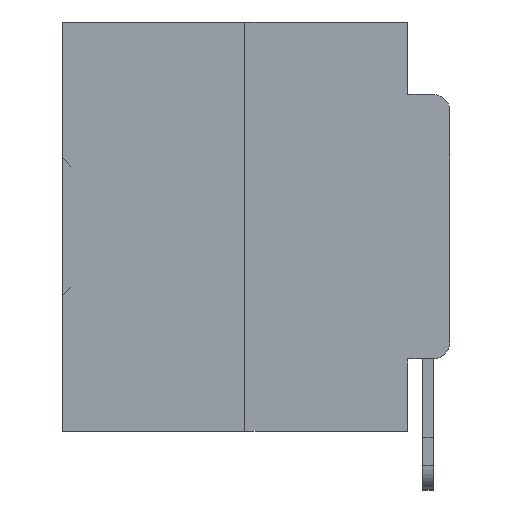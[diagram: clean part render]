
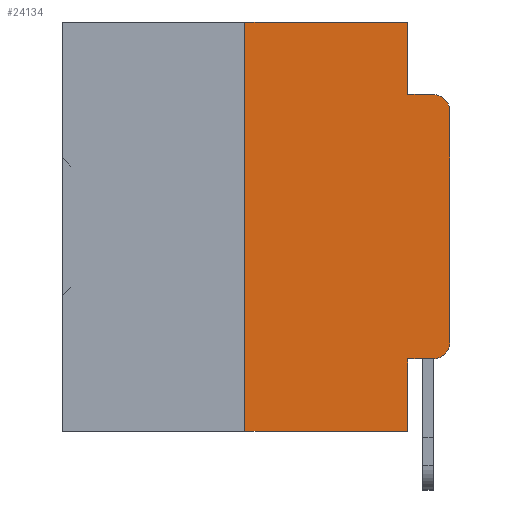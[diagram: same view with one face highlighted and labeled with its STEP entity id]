
A CAD part, left-side view. The second image highlights one B-rep face of the part: STEP entity #24134.
In plain terms, the highlighted planar face has unit normal (-1, 0, 0).
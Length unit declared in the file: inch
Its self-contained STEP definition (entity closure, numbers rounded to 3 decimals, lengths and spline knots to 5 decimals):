
#579 = ORIENTED_EDGE ( 'NONE', *, *, #16643, .T. ) ;
#754 = VERTEX_POINT ( 'NONE', #13273 ) ;
#968 = VECTOR ( 'NONE', #29545, 39.37008 ) ;
#1778 = VECTOR ( 'NONE', #3803, 39.37008 ) ;
#1877 = VECTOR ( 'NONE', #25889, 39.37008 ) ;
#2191 = CARTESIAN_POINT ( 'NONE',  ( 0., 0.051, 0. ) ) ;
#2324 = VERTEX_POINT ( 'NONE', #4209 ) ;
#2405 = EDGE_CURVE ( 'NONE', #12873, #13438, #32362, .T. ) ;
#2532 = EDGE_LOOP ( 'NONE', ( #579, #15423, #14845, #15844, #15766, #16718, #16315, #17418, #17161, #17482 ) ) ;
#3803 = DIRECTION ( 'NONE',  ( 0., -1., 0. ) ) ;
#3899 = VECTOR ( 'NONE', #19659, 39.37008 ) ;
#3977 = DIRECTION ( 'NONE',  ( 0., -1., 0. ) ) ;
#4209 = CARTESIAN_POINT ( 'NONE',  ( 0., 0.051, -0.4115 ) ) ;
#4798 = LINE ( 'NONE', #2191, #3899 ) ;
#5449 = CARTESIAN_POINT ( 'NONE',  ( 0., 0., 0. ) ) ;
#6075 = VERTEX_POINT ( 'NONE', #23513 ) ;
#6260 = DIRECTION ( 'NONE',  ( 1., 0., 0. ) ) ;
#7177 = VECTOR ( 'NONE', #3977, 39.37008 ) ;
#8425 = VECTOR ( 'NONE', #27502, 39.37008 ) ;
#8577 = VECTOR ( 'NONE', #21171, 39.37008 ) ;
#8808 = EDGE_CURVE ( 'NONE', #6075, #33764, #11815, .T. ) ;
#9530 = EDGE_CURVE ( 'NONE', #2324, #21305, #24114, .T. ) ;
#9562 = DIRECTION ( 'NONE',  ( 0., -1., 0. ) ) ;
#9589 = VERTEX_POINT ( 'NONE', #21438 ) ;
#9843 = CARTESIAN_POINT ( 'NONE',  ( 0., 0.051, -0.0885 ) ) ;
#9924 = CARTESIAN_POINT ( 'NONE',  ( 0., 0., -0.3915 ) ) ;
#10017 = CARTESIAN_POINT ( 'NONE',  ( 0., 0.25, 0. ) ) ;
#11717 = VERTEX_POINT ( 'NONE', #37247 ) ;
#11815 = CIRCLE ( 'NONE', #16608, 0.02 ) ;
#12084 = CARTESIAN_POINT ( 'NONE',  ( 0., 0.473, 0. ) ) ;
#12873 = VERTEX_POINT ( 'NONE', #19402 ) ;
#13273 = CARTESIAN_POINT ( 'NONE',  ( 0., 0.25, -0.5 ) ) ;
#13438 = VERTEX_POINT ( 'NONE', #9924 ) ;
#13723 = DIRECTION ( 'NONE',  ( -1., 0., 0. ) ) ;
#14128 = LINE ( 'NONE', #27052, #15959 ) ;
#14740 = VERTEX_POINT ( 'NONE', #27694 ) ;
#14845 = ORIENTED_EDGE ( 'NONE', *, *, #19133, .F. ) ;
#14929 = CARTESIAN_POINT ( 'NONE',  ( 0., 0.473, 0. ) ) ;
#15423 = ORIENTED_EDGE ( 'NONE', *, *, #8808, .T. ) ;
#15766 = ORIENTED_EDGE ( 'NONE', *, *, #16737, .F. ) ;
#15773 = AXIS2_PLACEMENT_3D ( 'NONE', #14929, #6260, #26675 ) ;
#15844 = ORIENTED_EDGE ( 'NONE', *, *, #34959, .F. ) ;
#15959 = VECTOR ( 'NONE', #9562, 39.37008 ) ;
#16315 = ORIENTED_EDGE ( 'NONE', *, *, #29065, .T. ) ;
#16608 = AXIS2_PLACEMENT_3D ( 'NONE', #31173, #13723, #34128 ) ;
#16643 = EDGE_CURVE ( 'NONE', #13438, #6075, #35655, .T. ) ;
#16718 = ORIENTED_EDGE ( 'NONE', *, *, #21179, .F. ) ;
#16737 = EDGE_CURVE ( 'NONE', #11717, #14740, #30160, .T. ) ;
#17161 = ORIENTED_EDGE ( 'NONE', *, *, #17815, .T. ) ;
#17418 = ORIENTED_EDGE ( 'NONE', *, *, #9530, .F. ) ;
#17482 = ORIENTED_EDGE ( 'NONE', *, *, #2405, .T. ) ;
#17815 = EDGE_CURVE ( 'NONE', #2324, #12873, #14128, .T. ) ;
#19133 = EDGE_CURVE ( 'NONE', #9589, #33764, #23598, .T. ) ;
#19402 = CARTESIAN_POINT ( 'NONE',  ( 0., 0.02, -0.4115 ) ) ;
#19659 = DIRECTION ( 'NONE',  ( 0., 0., -1. ) ) ;
#21171 = DIRECTION ( 'NONE',  ( 0., 0., -1. ) ) ;
#21179 = EDGE_CURVE ( 'NONE', #754, #11717, #23951, .T. ) ;
#21305 = VERTEX_POINT ( 'NONE', #36710 ) ;
#21438 = CARTESIAN_POINT ( 'NONE',  ( 0., 0.051, -0.0885 ) ) ;
#23513 = CARTESIAN_POINT ( 'NONE',  ( 0., 0., -0.1085 ) ) ;
#23598 = LINE ( 'NONE', #9843, #7177 ) ;
#23727 = PLANE ( 'NONE',  #15773 ) ;
#23951 = LINE ( 'NONE', #10017, #8425 ) ;
#24042 = AXIS2_PLACEMENT_3D ( 'NONE', #36841, #36650, #36798 ) ;
#24114 = LINE ( 'NONE', #35722, #8577 ) ;
#24134 = ADVANCED_FACE ( 'NONE', ( #37346 ), #23727, .F. ) ;
#25095 = LINE ( 'NONE', #35816, #1778 ) ;
#25889 = DIRECTION ( 'NONE',  ( 0., 0., 1. ) ) ;
#26675 = DIRECTION ( 'NONE',  ( 0., 0., -1. ) ) ;
#27052 = CARTESIAN_POINT ( 'NONE',  ( 0., 0.051, -0.4115 ) ) ;
#27502 = DIRECTION ( 'NONE',  ( 0., 0., 1. ) ) ;
#27694 = CARTESIAN_POINT ( 'NONE',  ( 0., 0.051, 0. ) ) ;
#29065 = EDGE_CURVE ( 'NONE', #754, #21305, #25095, .T. ) ;
#29545 = DIRECTION ( 'NONE',  ( 0., -1., 0. ) ) ;
#30160 = LINE ( 'NONE', #12084, #968 ) ;
#31173 = CARTESIAN_POINT ( 'NONE',  ( 0., 0.02, -0.1085 ) ) ;
#32362 = CIRCLE ( 'NONE', #24042, 0.02 ) ;
#33070 = CARTESIAN_POINT ( 'NONE',  ( 0., 0.02, -0.0885 ) ) ;
#33764 = VERTEX_POINT ( 'NONE', #33070 ) ;
#34128 = DIRECTION ( 'NONE',  ( 0., 0., -1. ) ) ;
#34959 = EDGE_CURVE ( 'NONE', #14740, #9589, #4798, .T. ) ;
#35655 = LINE ( 'NONE', #5449, #1877 ) ;
#35722 = CARTESIAN_POINT ( 'NONE',  ( 0., 0.051, 0. ) ) ;
#35816 = CARTESIAN_POINT ( 'NONE',  ( 0., 0.473, -0.5 ) ) ;
#36650 = DIRECTION ( 'NONE',  ( -1., 0., 0. ) ) ;
#36710 = CARTESIAN_POINT ( 'NONE',  ( 0., 0.051, -0.5 ) ) ;
#36798 = DIRECTION ( 'NONE',  ( 0., 0., -1. ) ) ;
#36841 = CARTESIAN_POINT ( 'NONE',  ( 0., 0.02, -0.3915 ) ) ;
#37247 = CARTESIAN_POINT ( 'NONE',  ( 0., 0.25, 0. ) ) ;
#37346 = FACE_OUTER_BOUND ( 'NONE', #2532, .T. ) ;
